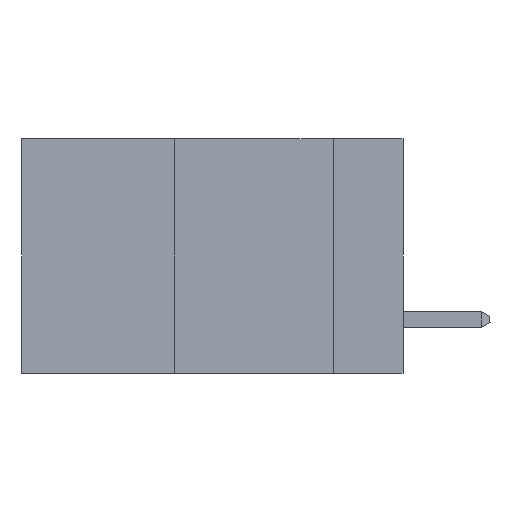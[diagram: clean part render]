
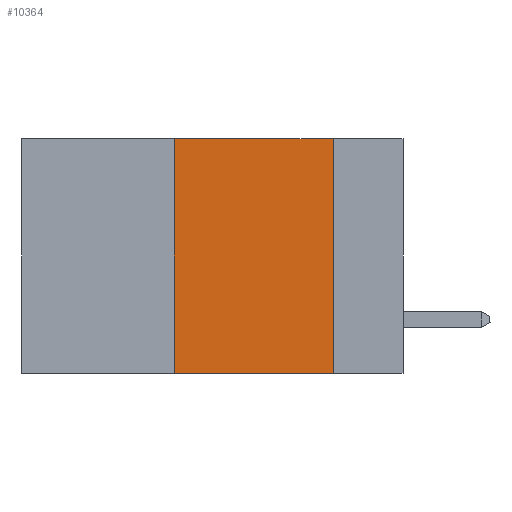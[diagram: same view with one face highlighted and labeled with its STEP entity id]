
A CAD part, left-side view. The second image highlights one B-rep face of the part: STEP entity #10364.
In plain terms, the highlighted planar face has unit normal (-1, 0, 0).
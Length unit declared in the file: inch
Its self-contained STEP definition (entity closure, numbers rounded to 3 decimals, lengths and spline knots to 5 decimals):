
#82 = EDGE_LOOP ( 'NONE', ( #10952, #8394, #1294, #4160 ) ) ;
#359 = CARTESIAN_POINT ( 'NONE',  ( 0., 0.6, -0.37 ) ) ;
#990 = DIRECTION ( 'NONE',  ( 0., 0., -1. ) ) ;
#1294 = ORIENTED_EDGE ( 'NONE', *, *, #3758, .F. ) ;
#1712 = AXIS2_PLACEMENT_3D ( 'NONE', #7344, #9543, #4236 ) ;
#3357 = LINE ( 'NONE', #8628, #12371 ) ;
#3377 = VERTEX_POINT ( 'NONE', #10920 ) ;
#3758 = EDGE_CURVE ( 'NONE', #3377, #8455, #13519, .T. ) ;
#4101 = EDGE_CURVE ( 'NONE', #3377, #13621, #8858, .T. ) ;
#4160 = ORIENTED_EDGE ( 'NONE', *, *, #4101, .T. ) ;
#4183 = PLANE ( 'NONE',  #1712 ) ;
#4221 = CARTESIAN_POINT ( 'NONE',  ( 0., 0.36, 0. ) ) ;
#4236 = DIRECTION ( 'NONE',  ( 0., 0., -1. ) ) ;
#5308 = DIRECTION ( 'NONE',  ( 0., 0., 1. ) ) ;
#5400 = DIRECTION ( 'NONE',  ( 0., -1., 0. ) ) ;
#6600 = VERTEX_POINT ( 'NONE', #10396 ) ;
#7344 = CARTESIAN_POINT ( 'NONE',  ( 0., 0.6, 0. ) ) ;
#7384 = EDGE_CURVE ( 'NONE', #6600, #13621, #8899, .T. ) ;
#7479 = FACE_OUTER_BOUND ( 'NONE', #82, .T. ) ;
#7497 = CARTESIAN_POINT ( 'NONE',  ( 0., 0.36, 0. ) ) ;
#8175 = EDGE_CURVE ( 'NONE', #8455, #6600, #3357, .T. ) ;
#8394 = ORIENTED_EDGE ( 'NONE', *, *, #8175, .F. ) ;
#8455 = VERTEX_POINT ( 'NONE', #7497 ) ;
#8628 = CARTESIAN_POINT ( 'NONE',  ( 0., 0.6, 0. ) ) ;
#8858 = LINE ( 'NONE', #359, #9184 ) ;
#8899 = LINE ( 'NONE', #12834, #12067 ) ;
#9184 = VECTOR ( 'NONE', #9853, 39.37008 ) ;
#9346 = VECTOR ( 'NONE', #5308, 39.37008 ) ;
#9543 = DIRECTION ( 'NONE',  ( 1., 0., 0. ) ) ;
#9853 = DIRECTION ( 'NONE',  ( 0., -1., 0. ) ) ;
#10364 = ADVANCED_FACE ( 'NONE', ( #7479 ), #4183, .F. ) ;
#10396 = CARTESIAN_POINT ( 'NONE',  ( 0., 0.11, 0. ) ) ;
#10920 = CARTESIAN_POINT ( 'NONE',  ( 0., 0.36, -0.37 ) ) ;
#10952 = ORIENTED_EDGE ( 'NONE', *, *, #7384, .F. ) ;
#12067 = VECTOR ( 'NONE', #990, 39.37008 ) ;
#12371 = VECTOR ( 'NONE', #5400, 39.37008 ) ;
#12834 = CARTESIAN_POINT ( 'NONE',  ( 0., 0.11, 0. ) ) ;
#13519 = LINE ( 'NONE', #4221, #9346 ) ;
#13621 = VERTEX_POINT ( 'NONE', #13704 ) ;
#13704 = CARTESIAN_POINT ( 'NONE',  ( 0., 0.11, -0.37 ) ) ;
